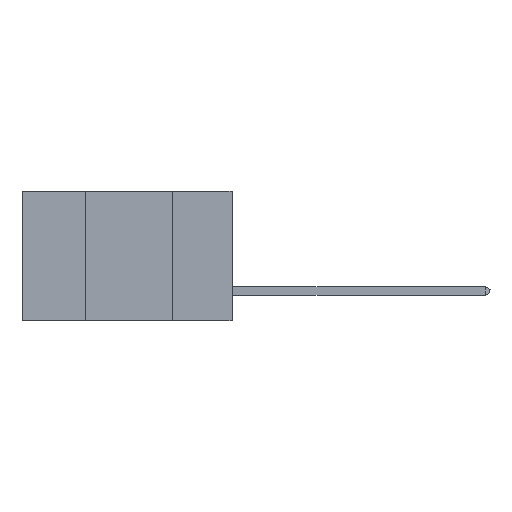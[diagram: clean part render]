
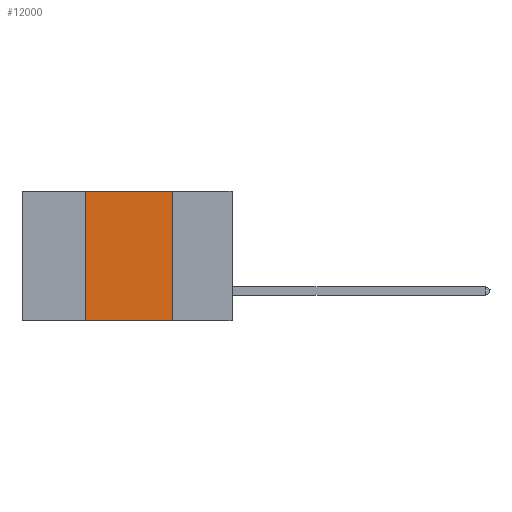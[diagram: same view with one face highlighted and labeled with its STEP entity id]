
A CAD part, left-side view. The second image highlights one B-rep face of the part: STEP entity #12000.
In plain terms, the highlighted planar face has unit normal (-1, 0, 0).
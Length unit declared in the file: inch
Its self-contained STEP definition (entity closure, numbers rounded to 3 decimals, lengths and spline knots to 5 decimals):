
#2030 = PLANE ( 'NONE',  #19958 ) ;
#5151 = CARTESIAN_POINT ( 'NONE',  ( 0., 0.17, 0. ) ) ;
#10099 = DIRECTION ( 'NONE',  ( 0., -1., 0. ) ) ;
#10150 = ORIENTED_EDGE ( 'NONE', *, *, #44249, .F. ) ;
#10302 = CARTESIAN_POINT ( 'NONE',  ( 0., 0.6, 0. ) ) ;
#10331 = VERTEX_POINT ( 'NONE', #29235 ) ;
#12000 = ADVANCED_FACE ( 'NONE', ( #40259 ), #2030, .F. ) ;
#14154 = CARTESIAN_POINT ( 'NONE',  ( 0., 0.42, -0.37 ) ) ;
#17373 = VECTOR ( 'NONE', #10099, 39.37008 ) ;
#17844 = VERTEX_POINT ( 'NONE', #43247 ) ;
#19824 = EDGE_CURVE ( 'NONE', #46919, #17844, #46354, .T. ) ;
#19958 = AXIS2_PLACEMENT_3D ( 'NONE', #29378, #37219, #46361 ) ;
#20038 = VECTOR ( 'NONE', #50846, 39.37008 ) ;
#20753 = VECTOR ( 'NONE', #49618, 39.37008 ) ;
#24026 = CARTESIAN_POINT ( 'NONE',  ( 0., 0.42, 0. ) ) ;
#26414 = LINE ( 'NONE', #34017, #31878 ) ;
#29235 = CARTESIAN_POINT ( 'NONE',  ( 0., 0.42, 0. ) ) ;
#29378 = CARTESIAN_POINT ( 'NONE',  ( 0., 0.6, 0. ) ) ;
#31344 = LINE ( 'NONE', #10302, #20753 ) ;
#31878 = VECTOR ( 'NONE', #49792, 39.37008 ) ;
#32224 = ORIENTED_EDGE ( 'NONE', *, *, #47507, .F. ) ;
#33948 = ORIENTED_EDGE ( 'NONE', *, *, #36757, .F. ) ;
#34017 = CARTESIAN_POINT ( 'NONE',  ( 0., 0.17, 0. ) ) ;
#34799 = ORIENTED_EDGE ( 'NONE', *, *, #19824, .T. ) ;
#36502 = EDGE_LOOP ( 'NONE', ( #32224, #33948, #10150, #34799 ) ) ;
#36757 = EDGE_CURVE ( 'NONE', #10331, #48376, #31344, .T. ) ;
#37219 = DIRECTION ( 'NONE',  ( 1., 0., 0. ) ) ;
#37733 = CARTESIAN_POINT ( 'NONE',  ( 0., 0.6, -0.37 ) ) ;
#40259 = FACE_OUTER_BOUND ( 'NONE', #36502, .T. ) ;
#42820 = LINE ( 'NONE', #24026, #20038 ) ;
#43247 = CARTESIAN_POINT ( 'NONE',  ( 0., 0.17, -0.37 ) ) ;
#44249 = EDGE_CURVE ( 'NONE', #46919, #10331, #42820, .T. ) ;
#46354 = LINE ( 'NONE', #37733, #17373 ) ;
#46361 = DIRECTION ( 'NONE',  ( 0., 0., -1. ) ) ;
#46919 = VERTEX_POINT ( 'NONE', #14154 ) ;
#47507 = EDGE_CURVE ( 'NONE', #48376, #17844, #26414, .T. ) ;
#48376 = VERTEX_POINT ( 'NONE', #5151 ) ;
#49618 = DIRECTION ( 'NONE',  ( 0., -1., 0. ) ) ;
#49792 = DIRECTION ( 'NONE',  ( 0., 0., -1. ) ) ;
#50846 = DIRECTION ( 'NONE',  ( 0., 0., 1. ) ) ;
